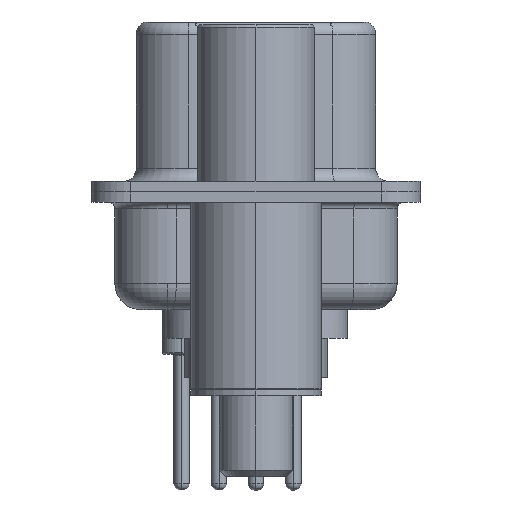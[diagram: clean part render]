
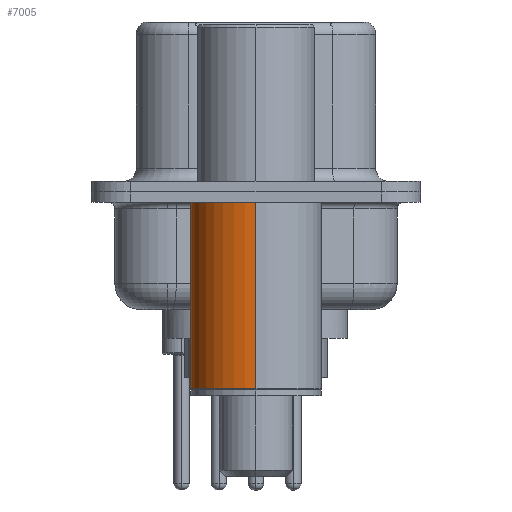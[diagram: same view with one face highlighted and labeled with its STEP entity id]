
A CAD part, left-side view. The second image highlights one B-rep face of the part: STEP entity #7005.
In plain terms, the highlighted cylindrical face has radius 2.5 mm (diameter 5 mm), a partial arc.
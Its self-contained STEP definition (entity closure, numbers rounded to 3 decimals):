
#158 = LINE ( 'NONE', #23704, #17712 ) ;
#290 = VERTEX_POINT ( 'NONE', #15589 ) ;
#1243 = ORIENTED_EDGE ( 'NONE', *, *, #25969, .F. ) ;
#1257 = CARTESIAN_POINT ( 'NONE',  ( 0., 0., -0.4 ) ) ;
#1483 = ORIENTED_EDGE ( 'NONE', *, *, #5406, .T. ) ;
#2549 = AXIS2_PLACEMENT_3D ( 'NONE', #1257, #17254, #3594 ) ;
#3594 = DIRECTION ( 'NONE',  ( 1., 0., 0. ) ) ;
#4019 = DIRECTION ( 'NONE',  ( 0., 0., 1. ) ) ;
#4357 = VERTEX_POINT ( 'NONE', #17546 ) ;
#5406 = EDGE_CURVE ( 'NONE', #290, #4357, #17660, .T. ) ;
#7005 = ADVANCED_FACE ( 'NONE', ( #10414 ), #21192, .T. ) ;
#7905 = CIRCLE ( 'NONE', #2549, 2.5 ) ;
#9911 = DIRECTION ( 'NONE',  ( 0., 0., 1. ) ) ;
#10414 = FACE_OUTER_BOUND ( 'NONE', #17054, .T. ) ;
#10967 = DIRECTION ( 'NONE',  ( 0., 0., 1. ) ) ;
#11214 = CARTESIAN_POINT ( 'NONE',  ( -2.5, 0., 0.581 ) ) ;
#12910 = VERTEX_POINT ( 'NONE', #17617 ) ;
#15437 = AXIS2_PLACEMENT_3D ( 'NONE', #19446, #26340, #17136 ) ;
#15589 = CARTESIAN_POINT ( 'NONE',  ( -2.5, 0., -7.525 ) ) ;
#16604 = AXIS2_PLACEMENT_3D ( 'NONE', #17675, #4019, #19994 ) ;
#16923 = VECTOR ( 'NONE', #10967, 1000. ) ;
#17054 = EDGE_LOOP ( 'NONE', ( #26754, #1483, #1243, #22846 ) ) ;
#17136 = DIRECTION ( 'NONE',  ( 1., 0., 0. ) ) ;
#17254 = DIRECTION ( 'NONE',  ( 0., 0., 1. ) ) ;
#17546 = CARTESIAN_POINT ( 'NONE',  ( -2.5, 0., -0.4 ) ) ;
#17617 = CARTESIAN_POINT ( 'NONE',  ( 2.5, 0., -0.4 ) ) ;
#17660 = LINE ( 'NONE', #11214, #16923 ) ;
#17675 = CARTESIAN_POINT ( 'NONE',  ( 0., 0., -7.525 ) ) ;
#17712 = VECTOR ( 'NONE', #9911, 1000. ) ;
#17737 = CIRCLE ( 'NONE', #16604, 2.5 ) ;
#19446 = CARTESIAN_POINT ( 'NONE',  ( 0., 0., 0.581 ) ) ;
#19994 = DIRECTION ( 'NONE',  ( 1., 0., 0. ) ) ;
#21192 = CYLINDRICAL_SURFACE ( 'NONE', #15437, 2.5 ) ;
#22309 = EDGE_CURVE ( 'NONE', #28660, #290, #17737, .T. ) ;
#22846 = ORIENTED_EDGE ( 'NONE', *, *, #22888, .F. ) ;
#22888 = EDGE_CURVE ( 'NONE', #28660, #12910, #158, .T. ) ;
#23704 = CARTESIAN_POINT ( 'NONE',  ( 2.5, 0., 0.581 ) ) ;
#25969 = EDGE_CURVE ( 'NONE', #12910, #4357, #7905, .T. ) ;
#26340 = DIRECTION ( 'NONE',  ( 0., 0., 1. ) ) ;
#26754 = ORIENTED_EDGE ( 'NONE', *, *, #22309, .T. ) ;
#27101 = CARTESIAN_POINT ( 'NONE',  ( 2.5, 0., -7.525 ) ) ;
#28660 = VERTEX_POINT ( 'NONE', #27101 ) ;
